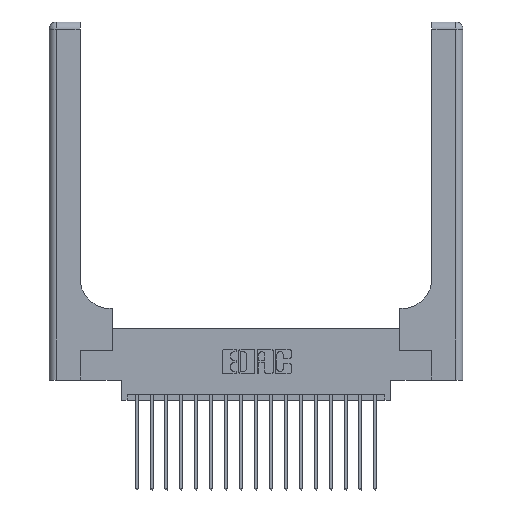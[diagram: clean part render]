
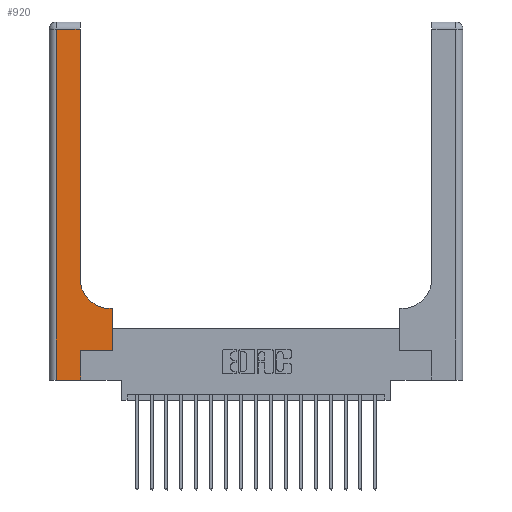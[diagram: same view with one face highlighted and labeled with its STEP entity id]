
A CAD part, top view. The second image highlights one B-rep face of the part: STEP entity #920.
In plain terms, the highlighted planar face has unit normal (0, 0, 1).
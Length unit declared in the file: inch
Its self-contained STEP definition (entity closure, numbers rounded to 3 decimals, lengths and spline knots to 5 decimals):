
#169 = ORIENTED_EDGE ( 'NONE', *, *, #1639, .T. ) ;
#920 = ADVANCED_FACE ( 'NONE', ( #18504 ), #11745, .F. ) ;
#1147 = CARTESIAN_POINT ( 'NONE',  ( 0.06, 2.94, 0.37 ) ) ;
#1153 = ORIENTED_EDGE ( 'NONE', *, *, #5412, .T. ) ;
#1394 = LINE ( 'NONE', #13068, #13156 ) ;
#1639 = EDGE_CURVE ( 'NONE', #4987, #7518, #7367, .T. ) ;
#2349 = CARTESIAN_POINT ( 'NONE',  ( 0.51, 0.85, 0.37 ) ) ;
#2523 = DIRECTION ( 'NONE',  ( -1., 0., 0. ) ) ;
#2578 = CARTESIAN_POINT ( 'NONE',  ( 0.26, 0.6, 0.37 ) ) ;
#2714 = EDGE_CURVE ( 'NONE', #16322, #6873, #9490, .T. ) ;
#2885 = CARTESIAN_POINT ( 'NONE',  ( 0.265, 0., 0.37 ) ) ;
#3200 = CARTESIAN_POINT ( 'NONE',  ( 0.528, 0.6, 0.37 ) ) ;
#3326 = EDGE_CURVE ( 'NONE', #6873, #4987, #19620, .T. ) ;
#3885 = DIRECTION ( 'NONE',  ( 1., 0., 0. ) ) ;
#3918 = DIRECTION ( 'NONE',  ( 1., 0., 0. ) ) ;
#4152 = DIRECTION ( 'NONE',  ( -1., 0., 0. ) ) ;
#4783 = ORIENTED_EDGE ( 'NONE', *, *, #8566, .T. ) ;
#4811 = LINE ( 'NONE', #11879, #16528 ) ;
#4987 = VERTEX_POINT ( 'NONE', #1147 ) ;
#5379 = VECTOR ( 'NONE', #11638, 39.37008 ) ;
#5412 = EDGE_CURVE ( 'NONE', #11386, #12959, #1394, .T. ) ;
#6439 = EDGE_CURVE ( 'NONE', #18942, #16322, #10083, .T. ) ;
#6873 = VERTEX_POINT ( 'NONE', #12322 ) ;
#7294 = CARTESIAN_POINT ( 'NONE',  ( 0.528, 0.25, 0.37 ) ) ;
#7367 = LINE ( 'NONE', #9046, #15937 ) ;
#7412 = AXIS2_PLACEMENT_3D ( 'NONE', #2349, #13092, #3918 ) ;
#7448 = CARTESIAN_POINT ( 'NONE',  ( 0.528, 0.25, 0.37 ) ) ;
#7499 = DIRECTION ( 'NONE',  ( 0., -1., 0. ) ) ;
#7518 = VERTEX_POINT ( 'NONE', #8006 ) ;
#8006 = CARTESIAN_POINT ( 'NONE',  ( 0.06, 0., 0.37 ) ) ;
#8566 = EDGE_CURVE ( 'NONE', #7518, #10989, #11182, .T. ) ;
#8897 = ORIENTED_EDGE ( 'NONE', *, *, #19177, .T. ) ;
#9046 = CARTESIAN_POINT ( 'NONE',  ( 0.06, 3., 0.37 ) ) ;
#9169 = DIRECTION ( 'NONE',  ( 1., 0., 0. ) ) ;
#9490 = LINE ( 'NONE', #14716, #5379 ) ;
#9785 = EDGE_LOOP ( 'NONE', ( #15071, #11492, #169, #4783, #8897, #1153, #13394, #17450, #9863 ) ) ;
#9854 = LINE ( 'NONE', #7448, #13862 ) ;
#9863 = ORIENTED_EDGE ( 'NONE', *, *, #6439, .T. ) ;
#10083 = CIRCLE ( 'NONE', #7412, 0.25 ) ;
#10699 = VECTOR ( 'NONE', #9169, 39.37008 ) ;
#10989 = VERTEX_POINT ( 'NONE', #2885 ) ;
#11181 = CARTESIAN_POINT ( 'NONE',  ( 0.51, 0.6, 0.37 ) ) ;
#11182 = LINE ( 'NONE', #16740, #10699 ) ;
#11386 = VERTEX_POINT ( 'NONE', #11490 ) ;
#11490 = CARTESIAN_POINT ( 'NONE',  ( 0.265, 0.25, 0.37 ) ) ;
#11492 = ORIENTED_EDGE ( 'NONE', *, *, #3326, .T. ) ;
#11498 = DIRECTION ( 'NONE',  ( -1., 0., 0. ) ) ;
#11502 = VECTOR ( 'NONE', #4152, 39.37008 ) ;
#11638 = DIRECTION ( 'NONE',  ( 0., 1., 0. ) ) ;
#11686 = DIRECTION ( 'NONE',  ( 0., 0., -1. ) ) ;
#11745 = PLANE ( 'NONE',  #12433 ) ;
#11782 = VERTEX_POINT ( 'NONE', #3200 ) ;
#11879 = CARTESIAN_POINT ( 'NONE',  ( 0.265, 0., 0.37 ) ) ;
#11947 = DIRECTION ( 'NONE',  ( 0., 1., 0. ) ) ;
#12146 = CARTESIAN_POINT ( 'NONE',  ( 0., 3., 0.37 ) ) ;
#12322 = CARTESIAN_POINT ( 'NONE',  ( 0.26, 2.94, 0.37 ) ) ;
#12433 = AXIS2_PLACEMENT_3D ( 'NONE', #12146, #11686, #11498 ) ;
#12959 = VERTEX_POINT ( 'NONE', #7294 ) ;
#13068 = CARTESIAN_POINT ( 'NONE',  ( 0.265, 0.25, 0.37 ) ) ;
#13092 = DIRECTION ( 'NONE',  ( 0., 0., -1. ) ) ;
#13156 = VECTOR ( 'NONE', #3885, 39.37008 ) ;
#13198 = CARTESIAN_POINT ( 'NONE',  ( 0., 2.94, 0.37 ) ) ;
#13394 = ORIENTED_EDGE ( 'NONE', *, *, #17994, .T. ) ;
#13479 = DIRECTION ( 'NONE',  ( 0., 1., 0. ) ) ;
#13680 = CARTESIAN_POINT ( 'NONE',  ( 0.26, 0.85, 0.37 ) ) ;
#13862 = VECTOR ( 'NONE', #13479, 39.37008 ) ;
#14716 = CARTESIAN_POINT ( 'NONE',  ( 0.26, 3., 0.37 ) ) ;
#15071 = ORIENTED_EDGE ( 'NONE', *, *, #2714, .T. ) ;
#15937 = VECTOR ( 'NONE', #7499, 39.37008 ) ;
#16035 = LINE ( 'NONE', #2578, #11502 ) ;
#16107 = VECTOR ( 'NONE', #2523, 39.37008 ) ;
#16322 = VERTEX_POINT ( 'NONE', #13680 ) ;
#16528 = VECTOR ( 'NONE', #11947, 39.37008 ) ;
#16740 = CARTESIAN_POINT ( 'NONE',  ( 0., 0., 0.37 ) ) ;
#17450 = ORIENTED_EDGE ( 'NONE', *, *, #19705, .T. ) ;
#17994 = EDGE_CURVE ( 'NONE', #12959, #11782, #9854, .T. ) ;
#18504 = FACE_OUTER_BOUND ( 'NONE', #9785, .T. ) ;
#18942 = VERTEX_POINT ( 'NONE', #11181 ) ;
#19177 = EDGE_CURVE ( 'NONE', #10989, #11386, #4811, .T. ) ;
#19620 = LINE ( 'NONE', #13198, #16107 ) ;
#19705 = EDGE_CURVE ( 'NONE', #11782, #18942, #16035, .T. ) ;
